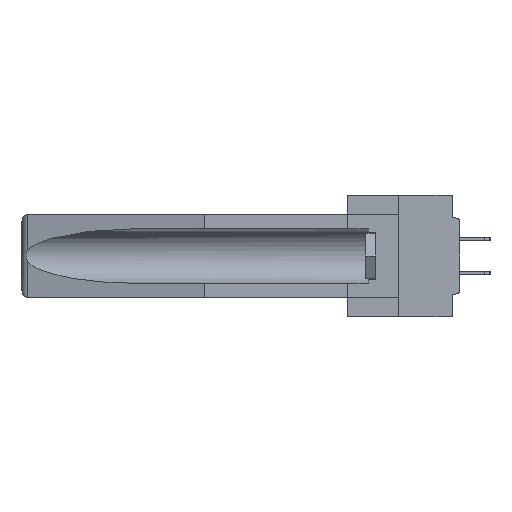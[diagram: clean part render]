
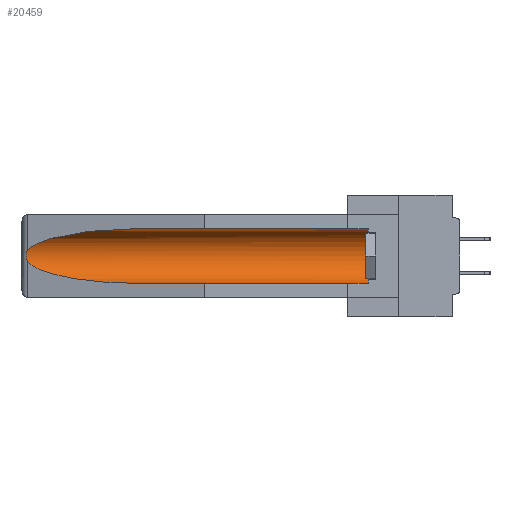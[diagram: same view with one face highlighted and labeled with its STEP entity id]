
A CAD part, left-side view. The second image highlights one B-rep face of the part: STEP entity #20459.
In plain terms, the highlighted cylindrical face has radius 2.857 mm (diameter 5.715 mm), a partial arc.
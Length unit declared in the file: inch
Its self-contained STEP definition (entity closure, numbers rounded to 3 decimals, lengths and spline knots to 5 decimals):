
#155 = EDGE_CURVE ( 'NONE', #35051, #15614, #31539, .T. ) ;
#588 = EDGE_CURVE ( 'NONE', #13706, #21312, #10838, .T. ) ;
#1505 = CARTESIAN_POINT ( 'NONE',  ( 0.155, 1.07973, -0.059 ) ) ;
#1871 = ORIENTED_EDGE ( 'NONE', *, *, #7509, .T. ) ;
#2034 = CARTESIAN_POINT ( 'NONE',  ( 0.26655, 1.53094, -0.18657 ) ) ;
#3461 = ORIENTED_EDGE ( 'NONE', *, *, #29242, .F. ) ;
#3998 = CARTESIAN_POINT ( 'NONE',  ( 0.155, 0.126, -0.1715 ) ) ;
#5128 = VECTOR ( 'NONE', #38713, 39.37008 ) ;
#6150 = AXIS2_PLACEMENT_3D ( 'NONE', #35535, #29011, #12772 ) ;
#7021 = FACE_OUTER_BOUND ( 'NONE', #12265, .T. ) ;
#7234 = DIRECTION ( 'NONE',  ( 0., 0., 1. ) ) ;
#7509 = EDGE_CURVE ( 'NONE', #16653, #35051, #20414, .T. ) ;
#8312 = CARTESIAN_POINT ( 'NONE',  ( 0.26537, 1.52718, -0.19328 ) ) ;
#8374 = CARTESIAN_POINT ( 'NONE',  ( 0.26597, 1.52961, -0.15275 ) ) ;
#8398 = VERTEX_POINT ( 'NONE', #22051 ) ;
#9924 = CARTESIAN_POINT ( 'NONE',  ( 0.21114, 1.30732, -0.059 ) ) ;
#9960 = ORIENTED_EDGE ( 'NONE', *, *, #41506, .T. ) ;
#9993 = CARTESIAN_POINT ( 'NONE',  ( 0.155, -0.30754, -0.059 ) ) ;
#10074 =( BOUNDED_CURVE ( )  B_SPLINE_CURVE ( 3, ( #8312, #37745, #11741, #28099 ),
 .UNSPECIFIED., .F., .F. ) 
 B_SPLINE_CURVE_WITH_KNOTS ( ( 4, 4 ),
 ( 0.1948, 1.5708 ),
 .UNSPECIFIED. ) 
 CURVE ( )  GEOMETRIC_REPRESENTATION_ITEM ( )  RATIONAL_B_SPLINE_CURVE ( ( 1., 0.848, 0.848, 1. ) ) 
 REPRESENTATION_ITEM ( '' )  );
#10838 = B_SPLINE_CURVE_WITH_KNOTS ( 'NONE', 3,
 ( #21646, #8374, #21507, #24893, #31430, #38091, #15235, #2034, #24747, #37810 ),
 .UNSPECIFIED., .F., .F.,
 ( 4, 2, 2, 2, 4 ),
 ( 0., 0.00029, 0.00058, 0.00087, 0.00117 ),
 .UNSPECIFIED. ) ;
#11741 = CARTESIAN_POINT ( 'NONE',  ( 0.21114, 1.30732, -0.284 ) ) ;
#12265 = EDGE_LOOP ( 'NONE', ( #29647, #32078, #9960, #3461, #1871, #23338 ) ) ;
#12772 = DIRECTION ( 'NONE',  ( 0., 0., 1. ) ) ;
#13706 = VERTEX_POINT ( 'NONE', #40876 ) ;
#14882 = VECTOR ( 'NONE', #29587, 39.37008 ) ;
#15235 = CARTESIAN_POINT ( 'NONE',  ( 0.2673, 1.53269, -0.17917 ) ) ;
#15614 = VERTEX_POINT ( 'NONE', #1505 ) ;
#16495 = CARTESIAN_POINT ( 'NONE',  ( 0.25451, 1.48313, -0.09465 ) ) ;
#16653 = VERTEX_POINT ( 'NONE', #25896 ) ;
#16917 = AXIS2_PLACEMENT_3D ( 'NONE', #3998, #26731, #7234 ) ;
#19779 = CARTESIAN_POINT ( 'NONE',  ( 0.155, -0.30754, -0.284 ) ) ;
#20398 = CARTESIAN_POINT ( 'NONE',  ( 0.26537, 1.52718, -0.19328 ) ) ;
#20414 = CIRCLE ( 'NONE', #16917, 0.1125 ) ;
#20459 = ADVANCED_FACE ( 'NONE', ( #7021 ), #21807, .F. ) ;
#21312 = VERTEX_POINT ( 'NONE', #20398 ) ;
#21507 = CARTESIAN_POINT ( 'NONE',  ( 0.26654, 1.53092, -0.15636 ) ) ;
#21646 = CARTESIAN_POINT ( 'NONE',  ( 0.26537, 1.52718, -0.14972 ) ) ;
#21807 = CYLINDRICAL_SURFACE ( 'NONE', #6150, 0.1125 ) ;
#22051 = CARTESIAN_POINT ( 'NONE',  ( 0.155, 1.07973, -0.284 ) ) ;
#22601 = CARTESIAN_POINT ( 'NONE',  ( 0.155, 1.07973, -0.059 ) ) ;
#23338 = ORIENTED_EDGE ( 'NONE', *, *, #155, .T. ) ;
#23544 = CARTESIAN_POINT ( 'NONE',  ( 0.155, 0.126, -0.059 ) ) ;
#23551 = LINE ( 'NONE', #19779, #14882 ) ;
#24747 = CARTESIAN_POINT ( 'NONE',  ( 0.26597, 1.5296, -0.19026 ) ) ;
#24893 = CARTESIAN_POINT ( 'NONE',  ( 0.2673, 1.5327, -0.16383 ) ) ;
#25896 = CARTESIAN_POINT ( 'NONE',  ( 0.155, 0.126, -0.284 ) ) ;
#26731 = DIRECTION ( 'NONE',  ( 0., -1., 0. ) ) ;
#27813 =( BOUNDED_CURVE ( )  B_SPLINE_CURVE ( 3, ( #22601, #9924, #16495, #32686 ),
 .UNSPECIFIED., .F., .F. ) 
 B_SPLINE_CURVE_WITH_KNOTS ( ( 4, 4 ),
 ( 4.71239, 6.08839 ),
 .UNSPECIFIED. ) 
 CURVE ( )  GEOMETRIC_REPRESENTATION_ITEM ( )  RATIONAL_B_SPLINE_CURVE ( ( 1., 0.848, 0.848, 1. ) ) 
 REPRESENTATION_ITEM ( '' )  );
#28099 = CARTESIAN_POINT ( 'NONE',  ( 0.155, 1.07973, -0.284 ) ) ;
#29011 = DIRECTION ( 'NONE',  ( 0., 1., 0. ) ) ;
#29242 = EDGE_CURVE ( 'NONE', #16653, #8398, #23551, .T. ) ;
#29587 = DIRECTION ( 'NONE',  ( 0., 1., 0. ) ) ;
#29647 = ORIENTED_EDGE ( 'NONE', *, *, #41176, .T. ) ;
#31430 = CARTESIAN_POINT ( 'NONE',  ( 0.2675, 1.53308, -0.16763 ) ) ;
#31539 = LINE ( 'NONE', #9993, #5128 ) ;
#32078 = ORIENTED_EDGE ( 'NONE', *, *, #588, .T. ) ;
#32686 = CARTESIAN_POINT ( 'NONE',  ( 0.26537, 1.52718, -0.14972 ) ) ;
#35051 = VERTEX_POINT ( 'NONE', #23544 ) ;
#35535 = CARTESIAN_POINT ( 'NONE',  ( 0.155, -0.30754, -0.1715 ) ) ;
#37745 = CARTESIAN_POINT ( 'NONE',  ( 0.25451, 1.48313, -0.24835 ) ) ;
#37810 = CARTESIAN_POINT ( 'NONE',  ( 0.26537, 1.52718, -0.19328 ) ) ;
#38091 = CARTESIAN_POINT ( 'NONE',  ( 0.2675, 1.53308, -0.17534 ) ) ;
#38713 = DIRECTION ( 'NONE',  ( 0., 1., 0. ) ) ;
#40876 = CARTESIAN_POINT ( 'NONE',  ( 0.26537, 1.52718, -0.14972 ) ) ;
#41176 = EDGE_CURVE ( 'NONE', #15614, #13706, #27813, .T. ) ;
#41506 = EDGE_CURVE ( 'NONE', #21312, #8398, #10074, .T. ) ;
